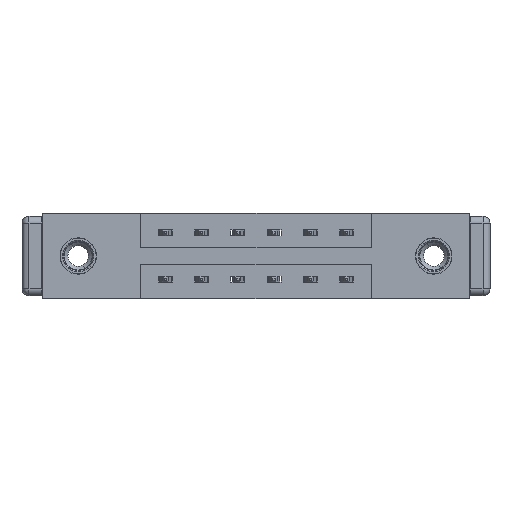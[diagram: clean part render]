
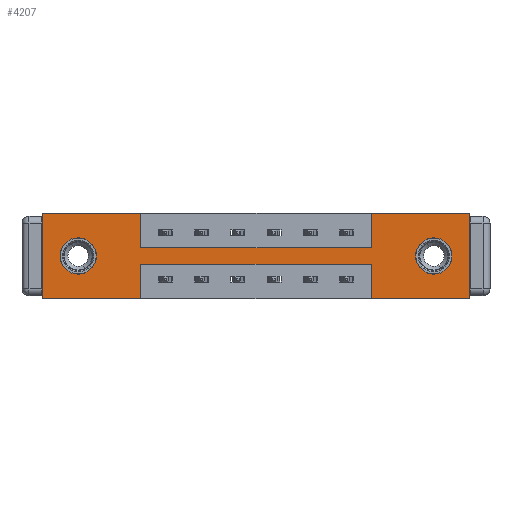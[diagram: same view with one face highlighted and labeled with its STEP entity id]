
A CAD part, front view. The second image highlights one B-rep face of the part: STEP entity #4207.
In plain terms, the highlighted planar face has unit normal (0, -1, 0).
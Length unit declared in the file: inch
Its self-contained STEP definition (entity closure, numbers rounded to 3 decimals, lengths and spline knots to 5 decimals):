
#32 = DIRECTION ( 'NONE',  ( -1., 0., 0. ) ) ;
#40 = AXIS2_PLACEMENT_3D ( 'NONE', #5902, #10588, #7701 ) ;
#84 = LINE ( 'NONE', #7569, #10457 ) ;
#99 = ORIENTED_EDGE ( 'NONE', *, *, #5985, .F. ) ;
#100 = VERTEX_POINT ( 'NONE', #3392 ) ;
#157 = ORIENTED_EDGE ( 'NONE', *, *, #2236, .T. ) ;
#310 = ORIENTED_EDGE ( 'NONE', *, *, #7222, .F. ) ;
#408 = VERTEX_POINT ( 'NONE', #8559 ) ;
#465 = EDGE_LOOP ( 'NONE', ( #99, #310, #1824, #4338, #9763, #3228, #7411, #1659, #10971, #9429, #10201, #2433 ) ) ;
#778 = FACE_BOUND ( 'NONE', #9945, .T. ) ;
#791 = CARTESIAN_POINT ( 'NONE',  ( 1.417, 0., -0.22 ) ) ;
#840 = LINE ( 'NONE', #9258, #2480 ) ;
#864 = VERTEX_POINT ( 'NONE', #11815 ) ;
#865 = VECTOR ( 'NONE', #7297, 39.37008 ) ;
#1128 = CARTESIAN_POINT ( 'NONE',  ( 0., 0., -0.37 ) ) ;
#1220 = DIRECTION ( 'NONE',  ( 0., 0., -1. ) ) ;
#1313 = DIRECTION ( 'NONE',  ( 0., 0., -1. ) ) ;
#1423 = VERTEX_POINT ( 'NONE', #2729 ) ;
#1443 = VERTEX_POINT ( 'NONE', #6346 ) ;
#1659 = ORIENTED_EDGE ( 'NONE', *, *, #6425, .F. ) ;
#1729 = CIRCLE ( 'NONE', #40, 0.078 ) ;
#1824 = ORIENTED_EDGE ( 'NONE', *, *, #7745, .F. ) ;
#1863 = AXIS2_PLACEMENT_3D ( 'NONE', #8374, #10285, #2914 ) ;
#1996 = CARTESIAN_POINT ( 'NONE',  ( 0.425, 0., -0.22 ) ) ;
#2037 = DIRECTION ( 'NONE',  ( -1., 0., 0. ) ) ;
#2175 = LINE ( 'NONE', #1996, #3355 ) ;
#2236 = EDGE_CURVE ( 'NONE', #8541, #10810, #5896, .T. ) ;
#2324 = CARTESIAN_POINT ( 'NONE',  ( 1.687, 0., -0.185 ) ) ;
#2433 = ORIENTED_EDGE ( 'NONE', *, *, #5541, .F. ) ;
#2480 = VECTOR ( 'NONE', #6600, 39.37008 ) ;
#2495 = DIRECTION ( 'NONE',  ( 0., 0., -1. ) ) ;
#2638 = CARTESIAN_POINT ( 'NONE',  ( 0.425, 0., -0.37 ) ) ;
#2729 = CARTESIAN_POINT ( 'NONE',  ( 0.155, 0., -0.263 ) ) ;
#2914 = DIRECTION ( 'NONE',  ( 0., 0., -1. ) ) ;
#3058 = PLANE ( 'NONE',  #8916 ) ;
#3147 = CARTESIAN_POINT ( 'NONE',  ( 0.155, 0., -0.185 ) ) ;
#3228 = ORIENTED_EDGE ( 'NONE', *, *, #7161, .F. ) ;
#3273 = DIRECTION ( 'NONE',  ( 1., 0., 0. ) ) ;
#3293 = VERTEX_POINT ( 'NONE', #5617 ) ;
#3355 = VECTOR ( 'NONE', #2037, 39.37008 ) ;
#3392 = CARTESIAN_POINT ( 'NONE',  ( 1.842, 0., -0.37 ) ) ;
#3409 = CIRCLE ( 'NONE', #10011, 0.078 ) ;
#3471 = LINE ( 'NONE', #9369, #5051 ) ;
#3575 = VERTEX_POINT ( 'NONE', #5096 ) ;
#3709 = CARTESIAN_POINT ( 'NONE',  ( 0.425, 0., 0. ) ) ;
#3745 = CARTESIAN_POINT ( 'NONE',  ( 0.425, 0., 0. ) ) ;
#3979 = CARTESIAN_POINT ( 'NONE',  ( 0., 0., 0. ) ) ;
#3999 = LINE ( 'NONE', #11532, #4304 ) ;
#4199 = ORIENTED_EDGE ( 'NONE', *, *, #6206, .T. ) ;
#4207 = ADVANCED_FACE ( 'NONE', ( #9068, #778, #6283 ), #3058, .T. ) ;
#4304 = VECTOR ( 'NONE', #7749, 39.37008 ) ;
#4338 = ORIENTED_EDGE ( 'NONE', *, *, #9247, .F. ) ;
#4403 = VERTEX_POINT ( 'NONE', #791 ) ;
#4979 = CARTESIAN_POINT ( 'NONE',  ( 1.842, 0., 0. ) ) ;
#5004 = VECTOR ( 'NONE', #5396, 39.37008 ) ;
#5051 = VECTOR ( 'NONE', #11358, 39.37008 ) ;
#5096 = CARTESIAN_POINT ( 'NONE',  ( 0.155, 0., -0.107 ) ) ;
#5223 = DIRECTION ( 'NONE',  ( 0., 1., 0. ) ) ;
#5396 = DIRECTION ( 'NONE',  ( 0., 0., -1. ) ) ;
#5444 = CARTESIAN_POINT ( 'NONE',  ( 0., 0., 0. ) ) ;
#5541 = EDGE_CURVE ( 'NONE', #11206, #864, #6712, .T. ) ;
#5617 = CARTESIAN_POINT ( 'NONE',  ( 1.417, 0., -0.37 ) ) ;
#5810 = DIRECTION ( 'NONE',  ( 1., 0., 0. ) ) ;
#5896 = CIRCLE ( 'NONE', #1863, 0.078 ) ;
#5902 = CARTESIAN_POINT ( 'NONE',  ( 0.155, 0., -0.185 ) ) ;
#5967 = VECTOR ( 'NONE', #3273, 39.37008 ) ;
#5985 = EDGE_CURVE ( 'NONE', #8983, #11206, #10512, .T. ) ;
#6206 = EDGE_CURVE ( 'NONE', #3575, #1423, #6995, .T. ) ;
#6283 = FACE_OUTER_BOUND ( 'NONE', #465, .T. ) ;
#6346 = CARTESIAN_POINT ( 'NONE',  ( 0.425, 0., -0.15 ) ) ;
#6425 = EDGE_CURVE ( 'NONE', #1443, #12101, #8433, .T. ) ;
#6600 = DIRECTION ( 'NONE',  ( 0., 0., 1. ) ) ;
#6602 = LINE ( 'NONE', #8530, #10139 ) ;
#6712 = LINE ( 'NONE', #9441, #10825 ) ;
#6995 = CIRCLE ( 'NONE', #11301, 0.078 ) ;
#7038 = EDGE_LOOP ( 'NONE', ( #157, #8885 ) ) ;
#7161 = EDGE_CURVE ( 'NONE', #408, #10036, #11676, .T. ) ;
#7222 = EDGE_CURVE ( 'NONE', #4403, #8983, #2175, .T. ) ;
#7297 = DIRECTION ( 'NONE',  ( 1., 0., 0. ) ) ;
#7302 = CARTESIAN_POINT ( 'NONE',  ( 0.425, 0., -0.37 ) ) ;
#7342 = ORIENTED_EDGE ( 'NONE', *, *, #8754, .T. ) ;
#7411 = ORIENTED_EDGE ( 'NONE', *, *, #8581, .F. ) ;
#7569 = CARTESIAN_POINT ( 'NONE',  ( 1.417, 0., -0.37 ) ) ;
#7590 = DIRECTION ( 'NONE',  ( 0., -1., 0. ) ) ;
#7619 = VERTEX_POINT ( 'NONE', #3745 ) ;
#7701 = DIRECTION ( 'NONE',  ( 0., 0., 1. ) ) ;
#7716 = VECTOR ( 'NONE', #9269, 39.37008 ) ;
#7738 = CARTESIAN_POINT ( 'NONE',  ( 1.842, 0., 0. ) ) ;
#7745 = EDGE_CURVE ( 'NONE', #3293, #4403, #84, .T. ) ;
#7749 = DIRECTION ( 'NONE',  ( 0., 0., 1. ) ) ;
#7758 = VERTEX_POINT ( 'NONE', #3979 ) ;
#7802 = EDGE_CURVE ( 'NONE', #10036, #100, #10181, .T. ) ;
#8374 = CARTESIAN_POINT ( 'NONE',  ( 1.687, 0., -0.185 ) ) ;
#8433 = LINE ( 'NONE', #10109, #5967 ) ;
#8530 = CARTESIAN_POINT ( 'NONE',  ( 0., 0., 0. ) ) ;
#8533 = VECTOR ( 'NONE', #1313, 39.37008 ) ;
#8541 = VERTEX_POINT ( 'NONE', #9219 ) ;
#8559 = CARTESIAN_POINT ( 'NONE',  ( 1.417, 0., 0. ) ) ;
#8581 = EDGE_CURVE ( 'NONE', #12101, #408, #840, .T. ) ;
#8625 = LINE ( 'NONE', #3709, #5004 ) ;
#8754 = EDGE_CURVE ( 'NONE', #1423, #3575, #1729, .T. ) ;
#8885 = ORIENTED_EDGE ( 'NONE', *, *, #11905, .T. ) ;
#8916 = AXIS2_PLACEMENT_3D ( 'NONE', #1128, #7590, #1220 ) ;
#8983 = VERTEX_POINT ( 'NONE', #11694 ) ;
#9068 = FACE_BOUND ( 'NONE', #7038, .T. ) ;
#9219 = CARTESIAN_POINT ( 'NONE',  ( 1.687, 0., -0.107 ) ) ;
#9247 = EDGE_CURVE ( 'NONE', #100, #3293, #3471, .T. ) ;
#9258 = CARTESIAN_POINT ( 'NONE',  ( 1.417, 0., 0. ) ) ;
#9269 = DIRECTION ( 'NONE',  ( 0., 0., -1. ) ) ;
#9369 = CARTESIAN_POINT ( 'NONE',  ( 0., 0., -0.37 ) ) ;
#9429 = ORIENTED_EDGE ( 'NONE', *, *, #10207, .F. ) ;
#9441 = CARTESIAN_POINT ( 'NONE',  ( 0., 0., -0.37 ) ) ;
#9638 = DIRECTION ( 'NONE',  ( 0., 1., 0. ) ) ;
#9763 = ORIENTED_EDGE ( 'NONE', *, *, #7802, .F. ) ;
#9945 = EDGE_LOOP ( 'NONE', ( #4199, #7342 ) ) ;
#10011 = AXIS2_PLACEMENT_3D ( 'NONE', #2324, #5223, #2495 ) ;
#10036 = VERTEX_POINT ( 'NONE', #7738 ) ;
#10037 = CARTESIAN_POINT ( 'NONE',  ( 1.417, 0., -0.15 ) ) ;
#10109 = CARTESIAN_POINT ( 'NONE',  ( 0.425, 0., -0.15 ) ) ;
#10139 = VECTOR ( 'NONE', #5810, 39.37008 ) ;
#10181 = LINE ( 'NONE', #4979, #8533 ) ;
#10201 = ORIENTED_EDGE ( 'NONE', *, *, #10882, .F. ) ;
#10207 = EDGE_CURVE ( 'NONE', #7758, #7619, #6602, .T. ) ;
#10285 = DIRECTION ( 'NONE',  ( 0., 1., 0. ) ) ;
#10325 = DIRECTION ( 'NONE',  ( 0., 0., 1. ) ) ;
#10457 = VECTOR ( 'NONE', #10325, 39.37008 ) ;
#10512 = LINE ( 'NONE', #2638, #7716 ) ;
#10588 = DIRECTION ( 'NONE',  ( 0., 1., 0. ) ) ;
#10595 = CARTESIAN_POINT ( 'NONE',  ( 1.687, 0., -0.263 ) ) ;
#10645 = DIRECTION ( 'NONE',  ( 0., 0., 1. ) ) ;
#10810 = VERTEX_POINT ( 'NONE', #10595 ) ;
#10825 = VECTOR ( 'NONE', #32, 39.37008 ) ;
#10882 = EDGE_CURVE ( 'NONE', #864, #7758, #3999, .T. ) ;
#10971 = ORIENTED_EDGE ( 'NONE', *, *, #11624, .F. ) ;
#11206 = VERTEX_POINT ( 'NONE', #7302 ) ;
#11301 = AXIS2_PLACEMENT_3D ( 'NONE', #3147, #9638, #10645 ) ;
#11358 = DIRECTION ( 'NONE',  ( -1., 0., 0. ) ) ;
#11532 = CARTESIAN_POINT ( 'NONE',  ( 0., 0., 0. ) ) ;
#11624 = EDGE_CURVE ( 'NONE', #7619, #1443, #8625, .T. ) ;
#11676 = LINE ( 'NONE', #5444, #865 ) ;
#11694 = CARTESIAN_POINT ( 'NONE',  ( 0.425, 0., -0.22 ) ) ;
#11815 = CARTESIAN_POINT ( 'NONE',  ( 0., 0., -0.37 ) ) ;
#11905 = EDGE_CURVE ( 'NONE', #10810, #8541, #3409, .T. ) ;
#12101 = VERTEX_POINT ( 'NONE', #10037 ) ;
